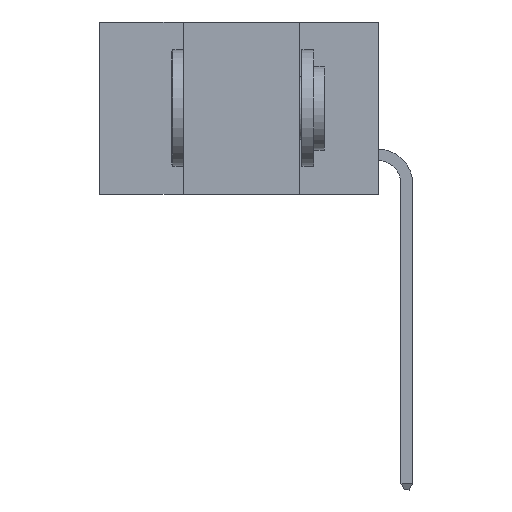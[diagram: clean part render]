
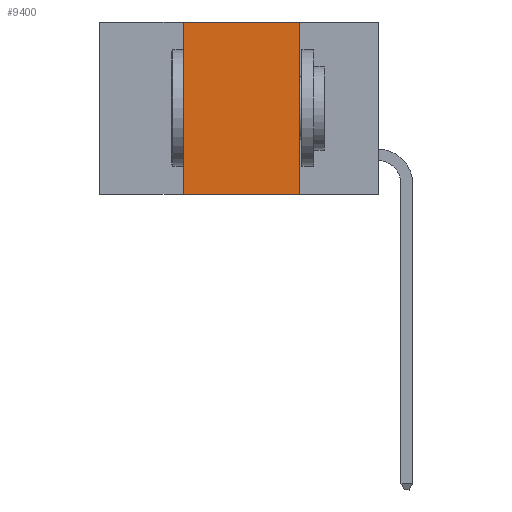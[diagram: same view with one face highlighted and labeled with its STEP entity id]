
A CAD part, left-side view. The second image highlights one B-rep face of the part: STEP entity #9400.
In plain terms, the highlighted planar face has unit normal (-1, 0, 0).
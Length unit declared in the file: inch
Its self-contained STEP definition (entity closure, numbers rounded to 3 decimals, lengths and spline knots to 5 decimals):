
#513 = LINE ( 'NONE', #8461, #787 ) ;
#646 = VERTEX_POINT ( 'NONE', #4316 ) ;
#787 = VECTOR ( 'NONE', #8703, 39.37008 ) ;
#989 = CARTESIAN_POINT ( 'NONE',  ( 0., 0.17, -0.37 ) ) ;
#1072 = EDGE_LOOP ( 'NONE', ( #2477, #9158, #3040, #10334 ) ) ;
#1654 = VERTEX_POINT ( 'NONE', #5605 ) ;
#2041 = EDGE_CURVE ( 'NONE', #1654, #6680, #513, .T. ) ;
#2423 = LINE ( 'NONE', #9694, #8431 ) ;
#2477 = ORIENTED_EDGE ( 'NONE', *, *, #3459, .F. ) ;
#2767 = DIRECTION ( 'NONE',  ( 0., 0., -1. ) ) ;
#2969 = FACE_OUTER_BOUND ( 'NONE', #1072, .T. ) ;
#2973 = VERTEX_POINT ( 'NONE', #989 ) ;
#2983 = LINE ( 'NONE', #5586, #7122 ) ;
#3040 = ORIENTED_EDGE ( 'NONE', *, *, #2041, .F. ) ;
#3063 = EDGE_CURVE ( 'NONE', #6680, #646, #2423, .T. ) ;
#3459 = EDGE_CURVE ( 'NONE', #646, #2973, #2983, .T. ) ;
#3584 = EDGE_CURVE ( 'NONE', #1654, #2973, #8176, .T. ) ;
#3933 = VECTOR ( 'NONE', #4151, 39.37008 ) ;
#4151 = DIRECTION ( 'NONE',  ( 0., -1., 0. ) ) ;
#4156 = DIRECTION ( 'NONE',  ( 0., -1., 0. ) ) ;
#4316 = CARTESIAN_POINT ( 'NONE',  ( 0., 0.17, 0. ) ) ;
#4416 = DIRECTION ( 'NONE',  ( 0., 0., -1. ) ) ;
#4426 = DIRECTION ( 'NONE',  ( 1., 0., 0. ) ) ;
#5175 = CARTESIAN_POINT ( 'NONE',  ( 0., 0.6, 0. ) ) ;
#5586 = CARTESIAN_POINT ( 'NONE',  ( 0., 0.17, 0. ) ) ;
#5605 = CARTESIAN_POINT ( 'NONE',  ( 0., 0.42, -0.37 ) ) ;
#5730 = PLANE ( 'NONE',  #8869 ) ;
#6450 = CARTESIAN_POINT ( 'NONE',  ( 0., 0.42, 0. ) ) ;
#6680 = VERTEX_POINT ( 'NONE', #6450 ) ;
#7122 = VECTOR ( 'NONE', #2767, 39.37008 ) ;
#7492 = CARTESIAN_POINT ( 'NONE',  ( 0., 0.6, -0.37 ) ) ;
#8176 = LINE ( 'NONE', #7492, #3933 ) ;
#8431 = VECTOR ( 'NONE', #4156, 39.37008 ) ;
#8461 = CARTESIAN_POINT ( 'NONE',  ( 0., 0.42, 0. ) ) ;
#8703 = DIRECTION ( 'NONE',  ( 0., 0., 1. ) ) ;
#8869 = AXIS2_PLACEMENT_3D ( 'NONE', #5175, #4426, #4416 ) ;
#9158 = ORIENTED_EDGE ( 'NONE', *, *, #3063, .F. ) ;
#9400 = ADVANCED_FACE ( 'NONE', ( #2969 ), #5730, .F. ) ;
#9694 = CARTESIAN_POINT ( 'NONE',  ( 0., 0.6, 0. ) ) ;
#10334 = ORIENTED_EDGE ( 'NONE', *, *, #3584, .T. ) ;
